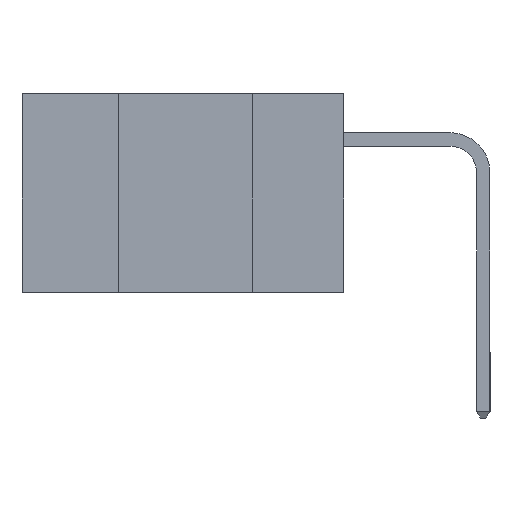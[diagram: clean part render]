
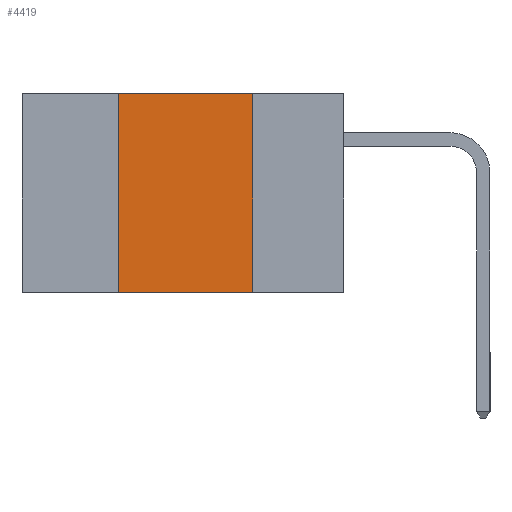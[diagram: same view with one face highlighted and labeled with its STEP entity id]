
A CAD part, left-side view. The second image highlights one B-rep face of the part: STEP entity #4419.
In plain terms, the highlighted planar face has unit normal (-1, 0, 0).
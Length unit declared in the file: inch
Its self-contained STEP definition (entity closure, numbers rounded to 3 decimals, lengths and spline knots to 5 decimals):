
#114 = DIRECTION ( 'NONE',  ( 0., -1., 0. ) ) ;
#1699 = LINE ( 'NONE', #1717, #2637 ) ;
#1717 = CARTESIAN_POINT ( 'NONE',  ( 0., 0.17, 0. ) ) ;
#1720 = CARTESIAN_POINT ( 'NONE',  ( 0., 0.42, -0.37 ) ) ;
#1771 = DIRECTION ( 'NONE',  ( 0., 0., -1. ) ) ;
#1890 = VECTOR ( 'NONE', #9821, 39.37008 ) ;
#2124 = DIRECTION ( 'NONE',  ( 0., -1., 0. ) ) ;
#2637 = VECTOR ( 'NONE', #1771, 39.37008 ) ;
#4419 = ADVANCED_FACE ( 'NONE', ( #6968 ), #12354, .F. ) ;
#4858 = LINE ( 'NONE', #11744, #14017 ) ;
#5047 = LINE ( 'NONE', #8843, #8437 ) ;
#5119 = CARTESIAN_POINT ( 'NONE',  ( 0., 0.42, 0. ) ) ;
#5127 = VERTEX_POINT ( 'NONE', #1720 ) ;
#5384 = EDGE_CURVE ( 'NONE', #5127, #6107, #4858, .T. ) ;
#5440 = EDGE_CURVE ( 'NONE', #9077, #12657, #5047, .T. ) ;
#6107 = VERTEX_POINT ( 'NONE', #7418 ) ;
#6968 = FACE_OUTER_BOUND ( 'NONE', #11052, .T. ) ;
#7179 = LINE ( 'NONE', #5119, #1890 ) ;
#7366 = ORIENTED_EDGE ( 'NONE', *, *, #9593, .F. ) ;
#7418 = CARTESIAN_POINT ( 'NONE',  ( 0., 0.17, -0.37 ) ) ;
#8437 = VECTOR ( 'NONE', #114, 39.37008 ) ;
#8843 = CARTESIAN_POINT ( 'NONE',  ( 0., 0.6, 0. ) ) ;
#9077 = VERTEX_POINT ( 'NONE', #14827 ) ;
#9593 = EDGE_CURVE ( 'NONE', #12657, #6107, #1699, .T. ) ;
#9821 = DIRECTION ( 'NONE',  ( 0., 0., 1. ) ) ;
#11052 = EDGE_LOOP ( 'NONE', ( #7366, #12336, #14548, #11721 ) ) ;
#11721 = ORIENTED_EDGE ( 'NONE', *, *, #5384, .T. ) ;
#11744 = CARTESIAN_POINT ( 'NONE',  ( 0., 0.6, -0.37 ) ) ;
#12336 = ORIENTED_EDGE ( 'NONE', *, *, #5440, .F. ) ;
#12354 = PLANE ( 'NONE',  #13561 ) ;
#12657 = VERTEX_POINT ( 'NONE', #13501 ) ;
#13463 = DIRECTION ( 'NONE',  ( 1., 0., 0. ) ) ;
#13501 = CARTESIAN_POINT ( 'NONE',  ( 0., 0.17, 0. ) ) ;
#13561 = AXIS2_PLACEMENT_3D ( 'NONE', #14477, #13463, #14525 ) ;
#13592 = EDGE_CURVE ( 'NONE', #5127, #9077, #7179, .T. ) ;
#14017 = VECTOR ( 'NONE', #2124, 39.37008 ) ;
#14477 = CARTESIAN_POINT ( 'NONE',  ( 0., 0.6, 0. ) ) ;
#14525 = DIRECTION ( 'NONE',  ( 0., 0., -1. ) ) ;
#14548 = ORIENTED_EDGE ( 'NONE', *, *, #13592, .F. ) ;
#14827 = CARTESIAN_POINT ( 'NONE',  ( 0., 0.42, 0. ) ) ;
